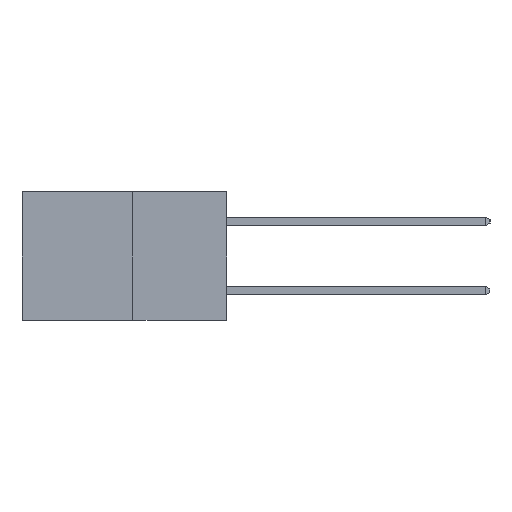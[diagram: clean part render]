
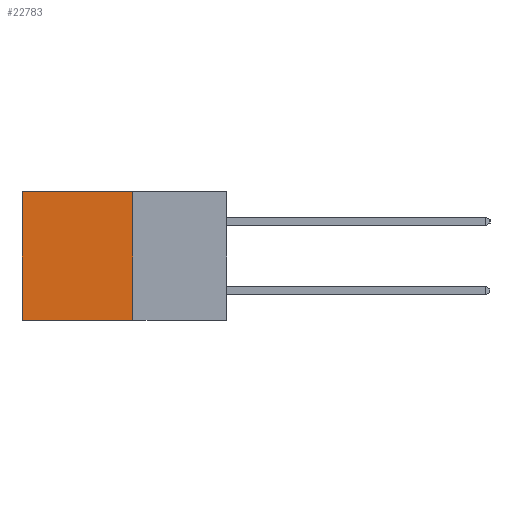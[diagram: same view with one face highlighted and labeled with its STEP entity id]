
A CAD part, left-side view. The second image highlights one B-rep face of the part: STEP entity #22783.
In plain terms, the highlighted planar face has unit normal (-1, 0, 0).
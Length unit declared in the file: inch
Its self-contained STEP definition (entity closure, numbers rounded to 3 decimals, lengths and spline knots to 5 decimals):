
#711 = CARTESIAN_POINT ( 'NONE',  ( 0.277, 0.27, -0.37 ) ) ;
#737 = LINE ( 'NONE', #21579, #11964 ) ;
#1753 = EDGE_CURVE ( 'NONE', #5348, #24087, #25856, .T. ) ;
#2521 = VERTEX_POINT ( 'NONE', #8978 ) ;
#3580 = EDGE_CURVE ( 'NONE', #28351, #2521, #737, .T. ) ;
#4211 = EDGE_CURVE ( 'NONE', #24087, #2521, #18977, .T. ) ;
#4574 = DIRECTION ( 'NONE',  ( 0., 0., -1. ) ) ;
#5348 = VERTEX_POINT ( 'NONE', #19990 ) ;
#5655 = ORIENTED_EDGE ( 'NONE', *, *, #28782, .F. ) ;
#5937 = FACE_OUTER_BOUND ( 'NONE', #8410, .T. ) ;
#6944 = VECTOR ( 'NONE', #4574, 39.37008 ) ;
#8260 = CARTESIAN_POINT ( 'NONE',  ( 0.277, 0.27, 0. ) ) ;
#8410 = EDGE_LOOP ( 'NONE', ( #15001, #12640, #5655, #28325 ) ) ;
#8978 = CARTESIAN_POINT ( 'NONE',  ( 0.277, 0.59, -0.37 ) ) ;
#9311 = DIRECTION ( 'NONE',  ( 0., 0., -1. ) ) ;
#11964 = VECTOR ( 'NONE', #19473, 39.37008 ) ;
#12640 = ORIENTED_EDGE ( 'NONE', *, *, #3580, .F. ) ;
#13762 = PLANE ( 'NONE',  #22515 ) ;
#13806 = VECTOR ( 'NONE', #19007, 39.37008 ) ;
#14823 = LINE ( 'NONE', #24764, #20149 ) ;
#15001 = ORIENTED_EDGE ( 'NONE', *, *, #4211, .T. ) ;
#15683 = DIRECTION ( 'NONE',  ( 0., 0., -1. ) ) ;
#16808 = CARTESIAN_POINT ( 'NONE',  ( 0.277, 0.59, -0.37 ) ) ;
#18977 = LINE ( 'NONE', #16808, #6944 ) ;
#19007 = DIRECTION ( 'NONE',  ( 0., 1., 0. ) ) ;
#19473 = DIRECTION ( 'NONE',  ( 0., 1., 0. ) ) ;
#19990 = CARTESIAN_POINT ( 'NONE',  ( 0.277, 0.27, 0. ) ) ;
#20149 = VECTOR ( 'NONE', #15683, 39.37008 ) ;
#20322 = CARTESIAN_POINT ( 'NONE',  ( 0.277, 0.59, 0. ) ) ;
#20581 = CARTESIAN_POINT ( 'NONE',  ( 0.277, 0.27, -0.37 ) ) ;
#21579 = CARTESIAN_POINT ( 'NONE',  ( 0.277, 0.27, -0.37 ) ) ;
#22515 = AXIS2_PLACEMENT_3D ( 'NONE', #20581, #22925, #9311 ) ;
#22783 = ADVANCED_FACE ( 'NONE', ( #5937 ), #13762, .F. ) ;
#22925 = DIRECTION ( 'NONE',  ( 1., 0., 0. ) ) ;
#24087 = VERTEX_POINT ( 'NONE', #20322 ) ;
#24764 = CARTESIAN_POINT ( 'NONE',  ( 0.277, 0.27, -0.37 ) ) ;
#25856 = LINE ( 'NONE', #8260, #13806 ) ;
#28325 = ORIENTED_EDGE ( 'NONE', *, *, #1753, .T. ) ;
#28351 = VERTEX_POINT ( 'NONE', #711 ) ;
#28782 = EDGE_CURVE ( 'NONE', #5348, #28351, #14823, .T. ) ;
